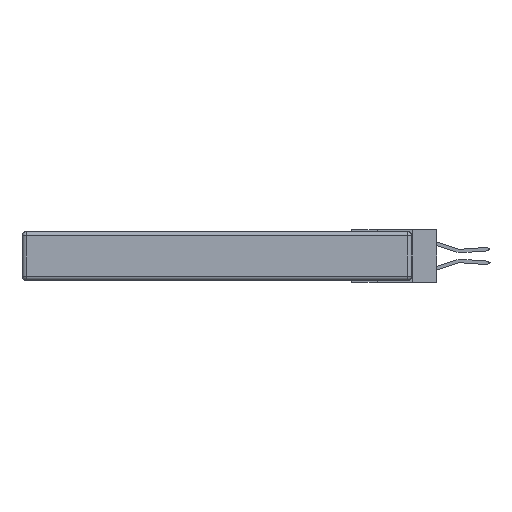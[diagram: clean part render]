
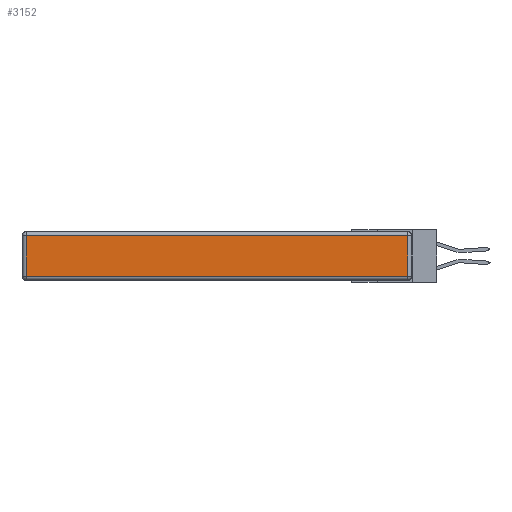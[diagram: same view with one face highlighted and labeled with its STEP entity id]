
A CAD part, left-side view. The second image highlights one B-rep face of the part: STEP entity #3152.
In plain terms, the highlighted planar face has unit normal (-1, 0, 0).
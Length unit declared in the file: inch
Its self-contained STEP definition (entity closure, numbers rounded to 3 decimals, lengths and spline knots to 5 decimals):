
#378 = DIRECTION ( 'NONE',  ( 0., 0., -1. ) ) ;
#843 = DIRECTION ( 'NONE',  ( 0., 1., 0. ) ) ;
#988 = CARTESIAN_POINT ( 'NONE',  ( 0., 0.03, -0.313 ) ) ;
#2483 = LINE ( 'NONE', #10857, #12893 ) ;
#2874 = EDGE_CURVE ( 'NONE', #8330, #10484, #17277, .T. ) ;
#3152 = ADVANCED_FACE ( 'NONE', ( #16242 ), #8324, .T. ) ;
#5041 = EDGE_CURVE ( 'NONE', #10484, #19006, #2483, .T. ) ;
#6437 = VECTOR ( 'NONE', #378, 39.37008 ) ;
#7672 = EDGE_CURVE ( 'NONE', #12346, #8330, #17027, .T. ) ;
#8324 = PLANE ( 'NONE',  #10873 ) ;
#8330 = VERTEX_POINT ( 'NONE', #988 ) ;
#8407 = CARTESIAN_POINT ( 'NONE',  ( 0., 2.72, -0.03 ) ) ;
#8917 = ORIENTED_EDGE ( 'NONE', *, *, #5041, .T. ) ;
#9026 = EDGE_LOOP ( 'NONE', ( #12328, #15608, #8917, #14634 ) ) ;
#9774 = LINE ( 'NONE', #9898, #6437 ) ;
#9898 = CARTESIAN_POINT ( 'NONE',  ( 0., 2.72, -0.343 ) ) ;
#10484 = VERTEX_POINT ( 'NONE', #17685 ) ;
#10857 = CARTESIAN_POINT ( 'NONE',  ( 0., 2.75, -0.03 ) ) ;
#10873 = AXIS2_PLACEMENT_3D ( 'NONE', #19928, #11826, #19785 ) ;
#10982 = CARTESIAN_POINT ( 'NONE',  ( 0., 0.03, -0.343 ) ) ;
#11657 = VECTOR ( 'NONE', #14702, 39.37008 ) ;
#11826 = DIRECTION ( 'NONE',  ( -1., 0., 0. ) ) ;
#12328 = ORIENTED_EDGE ( 'NONE', *, *, #7672, .T. ) ;
#12346 = VERTEX_POINT ( 'NONE', #19541 ) ;
#12893 = VECTOR ( 'NONE', #843, 39.37008 ) ;
#13291 = CARTESIAN_POINT ( 'NONE',  ( 0., 0., -0.313 ) ) ;
#14463 = VECTOR ( 'NONE', #19158, 39.37008 ) ;
#14634 = ORIENTED_EDGE ( 'NONE', *, *, #21120, .T. ) ;
#14702 = DIRECTION ( 'NONE',  ( 0., -1., 0. ) ) ;
#15608 = ORIENTED_EDGE ( 'NONE', *, *, #2874, .T. ) ;
#16242 = FACE_OUTER_BOUND ( 'NONE', #9026, .T. ) ;
#17027 = LINE ( 'NONE', #13291, #11657 ) ;
#17277 = LINE ( 'NONE', #10982, #14463 ) ;
#17685 = CARTESIAN_POINT ( 'NONE',  ( 0., 0.03, -0.03 ) ) ;
#19006 = VERTEX_POINT ( 'NONE', #8407 ) ;
#19158 = DIRECTION ( 'NONE',  ( 0., 0., 1. ) ) ;
#19541 = CARTESIAN_POINT ( 'NONE',  ( 0., 2.72, -0.313 ) ) ;
#19785 = DIRECTION ( 'NONE',  ( 0., 0., 1. ) ) ;
#19928 = CARTESIAN_POINT ( 'NONE',  ( 0., 0., -0.343 ) ) ;
#21120 = EDGE_CURVE ( 'NONE', #19006, #12346, #9774, .T. ) ;
